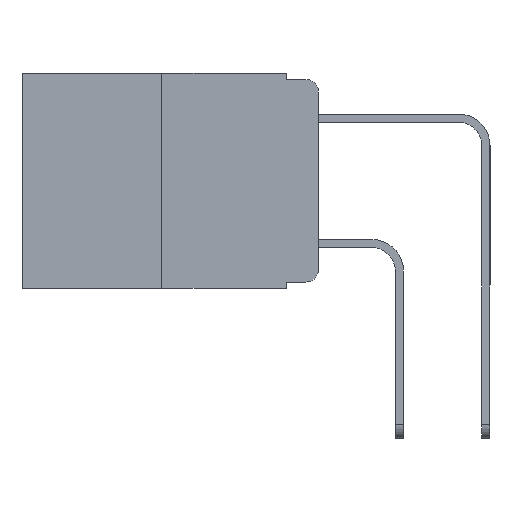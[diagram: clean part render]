
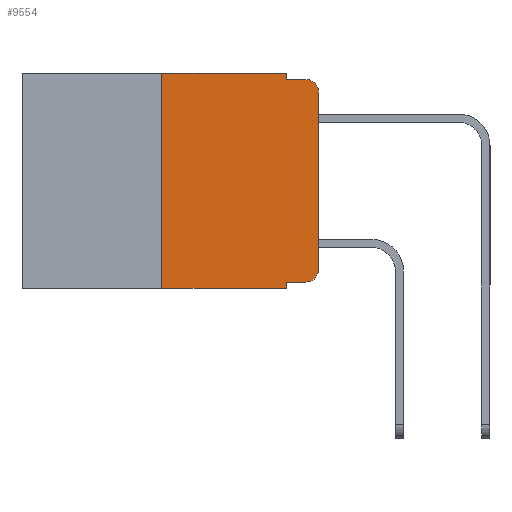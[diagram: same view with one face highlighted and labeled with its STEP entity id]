
A CAD part, left-side view. The second image highlights one B-rep face of the part: STEP entity #9554.
In plain terms, the highlighted planar face has unit normal (-1, 0, 0).
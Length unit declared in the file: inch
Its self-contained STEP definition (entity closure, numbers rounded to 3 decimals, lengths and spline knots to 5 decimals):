
#43 = CIRCLE ( 'NONE', #4933, 0.02 ) ;
#471 = VECTOR ( 'NONE', #12869, 39.37008 ) ;
#511 = LINE ( 'NONE', #546, #9162 ) ;
#546 = CARTESIAN_POINT ( 'NONE',  ( 0., 0.051, 0. ) ) ;
#586 = EDGE_CURVE ( 'NONE', #7244, #9654, #5994, .T. ) ;
#883 = EDGE_LOOP ( 'NONE', ( #1202, #3242, #4131, #4845, #13861, #3781, #10762, #4053, #4771, #5974 ) ) ;
#994 = LINE ( 'NONE', #8828, #6370 ) ;
#1027 = CARTESIAN_POINT ( 'NONE',  ( 0., 0.473, 0. ) ) ;
#1041 = FACE_OUTER_BOUND ( 'NONE', #883, .T. ) ;
#1073 = DIRECTION ( 'NONE',  ( -1., 0., 0. ) ) ;
#1202 = ORIENTED_EDGE ( 'NONE', *, *, #8927, .T. ) ;
#1535 = VECTOR ( 'NONE', #7794, 39.37008 ) ;
#1580 = EDGE_CURVE ( 'NONE', #11815, #4133, #994, .T. ) ;
#1731 = DIRECTION ( 'NONE',  ( 0., -1., 0. ) ) ;
#2060 = CARTESIAN_POINT ( 'NONE',  ( 0., 0.25, 0. ) ) ;
#2095 = CARTESIAN_POINT ( 'NONE',  ( 0., 0.02, -0.333 ) ) ;
#2253 = EDGE_CURVE ( 'NONE', #7244, #4133, #7221, .T. ) ;
#2478 = CARTESIAN_POINT ( 'NONE',  ( 0., 0.25, 0. ) ) ;
#2582 = DIRECTION ( 'NONE',  ( 0., -1., 0. ) ) ;
#2888 = CARTESIAN_POINT ( 'NONE',  ( 0., 0.051, 0. ) ) ;
#2957 = CARTESIAN_POINT ( 'NONE',  ( 0., 0.051, -0.01 ) ) ;
#3046 = VECTOR ( 'NONE', #2582, 39.37008 ) ;
#3075 = EDGE_CURVE ( 'NONE', #11815, #12192, #12897, .T. ) ;
#3242 = ORIENTED_EDGE ( 'NONE', *, *, #8228, .T. ) ;
#3290 = AXIS2_PLACEMENT_3D ( 'NONE', #7845, #1073, #9110 ) ;
#3630 = CARTESIAN_POINT ( 'NONE',  ( 0., 0.02, -0.313 ) ) ;
#3781 = ORIENTED_EDGE ( 'NONE', *, *, #3075, .F. ) ;
#4053 = ORIENTED_EDGE ( 'NONE', *, *, #2253, .F. ) ;
#4131 = ORIENTED_EDGE ( 'NONE', *, *, #6047, .F. ) ;
#4133 = VERTEX_POINT ( 'NONE', #7972 ) ;
#4358 = DIRECTION ( 'NONE',  ( 0., 0., -1. ) ) ;
#4361 = LINE ( 'NONE', #7532, #10392 ) ;
#4565 = EDGE_CURVE ( 'NONE', #12506, #7909, #511, .T. ) ;
#4759 = DIRECTION ( 'NONE',  ( 0., 0., -1. ) ) ;
#4771 = ORIENTED_EDGE ( 'NONE', *, *, #586, .T. ) ;
#4845 = ORIENTED_EDGE ( 'NONE', *, *, #4565, .F. ) ;
#4933 = AXIS2_PLACEMENT_3D ( 'NONE', #3630, #11081, #4759 ) ;
#5345 = DIRECTION ( 'NONE',  ( 1., 0., 0. ) ) ;
#5615 = AXIS2_PLACEMENT_3D ( 'NONE', #10623, #5345, #12590 ) ;
#5974 = ORIENTED_EDGE ( 'NONE', *, *, #13815, .T. ) ;
#5994 = LINE ( 'NONE', #13726, #3046 ) ;
#6047 = EDGE_CURVE ( 'NONE', #7909, #10761, #7122, .T. ) ;
#6370 = VECTOR ( 'NONE', #8811, 39.37008 ) ;
#6551 = CARTESIAN_POINT ( 'NONE',  ( 0., 0., -0.313 ) ) ;
#6608 = LINE ( 'NONE', #1027, #471 ) ;
#6825 = VERTEX_POINT ( 'NONE', #6551 ) ;
#7122 = LINE ( 'NONE', #2957, #12239 ) ;
#7221 = LINE ( 'NONE', #2888, #12319 ) ;
#7244 = VERTEX_POINT ( 'NONE', #7272 ) ;
#7272 = CARTESIAN_POINT ( 'NONE',  ( 0., 0.051, -0.333 ) ) ;
#7492 = CIRCLE ( 'NONE', #3290, 0.02 ) ;
#7532 = CARTESIAN_POINT ( 'NONE',  ( 0., 0., 0. ) ) ;
#7723 = CARTESIAN_POINT ( 'NONE',  ( 0., 0.051, 0. ) ) ;
#7794 = DIRECTION ( 'NONE',  ( 0., 0., 1. ) ) ;
#7845 = CARTESIAN_POINT ( 'NONE',  ( 0., 0.02, -0.03 ) ) ;
#7909 = VERTEX_POINT ( 'NONE', #11385 ) ;
#7972 = CARTESIAN_POINT ( 'NONE',  ( 0., 0.051, -0.343 ) ) ;
#8228 = EDGE_CURVE ( 'NONE', #13581, #10761, #7492, .T. ) ;
#8516 = EDGE_CURVE ( 'NONE', #12192, #12506, #6608, .T. ) ;
#8811 = DIRECTION ( 'NONE',  ( 0., -1., 0. ) ) ;
#8828 = CARTESIAN_POINT ( 'NONE',  ( 0., 0.473, -0.343 ) ) ;
#8927 = EDGE_CURVE ( 'NONE', #6825, #13581, #4361, .T. ) ;
#9110 = DIRECTION ( 'NONE',  ( 0., 0., -1. ) ) ;
#9162 = VECTOR ( 'NONE', #13332, 39.37008 ) ;
#9554 = ADVANCED_FACE ( 'NONE', ( #1041 ), #9609, .F. ) ;
#9609 = PLANE ( 'NONE',  #5615 ) ;
#9627 = DIRECTION ( 'NONE',  ( 0., 0., 1. ) ) ;
#9654 = VERTEX_POINT ( 'NONE', #2095 ) ;
#10392 = VECTOR ( 'NONE', #9627, 39.37008 ) ;
#10502 = CARTESIAN_POINT ( 'NONE',  ( 0., 0.25, -0.343 ) ) ;
#10623 = CARTESIAN_POINT ( 'NONE',  ( 0., 0.473, 0. ) ) ;
#10761 = VERTEX_POINT ( 'NONE', #12773 ) ;
#10762 = ORIENTED_EDGE ( 'NONE', *, *, #1580, .T. ) ;
#11081 = DIRECTION ( 'NONE',  ( -1., 0., 0. ) ) ;
#11385 = CARTESIAN_POINT ( 'NONE',  ( 0., 0.051, -0.01 ) ) ;
#11611 = CARTESIAN_POINT ( 'NONE',  ( 0., 0., -0.03 ) ) ;
#11815 = VERTEX_POINT ( 'NONE', #10502 ) ;
#12192 = VERTEX_POINT ( 'NONE', #2478 ) ;
#12239 = VECTOR ( 'NONE', #1731, 39.37008 ) ;
#12319 = VECTOR ( 'NONE', #4358, 39.37008 ) ;
#12506 = VERTEX_POINT ( 'NONE', #7723 ) ;
#12590 = DIRECTION ( 'NONE',  ( 0., 0., -1. ) ) ;
#12773 = CARTESIAN_POINT ( 'NONE',  ( 0., 0.02, -0.01 ) ) ;
#12869 = DIRECTION ( 'NONE',  ( 0., -1., 0. ) ) ;
#12897 = LINE ( 'NONE', #2060, #1535 ) ;
#13332 = DIRECTION ( 'NONE',  ( 0., 0., -1. ) ) ;
#13581 = VERTEX_POINT ( 'NONE', #11611 ) ;
#13726 = CARTESIAN_POINT ( 'NONE',  ( 0., 0.051, -0.333 ) ) ;
#13815 = EDGE_CURVE ( 'NONE', #9654, #6825, #43, .T. ) ;
#13861 = ORIENTED_EDGE ( 'NONE', *, *, #8516, .F. ) ;
